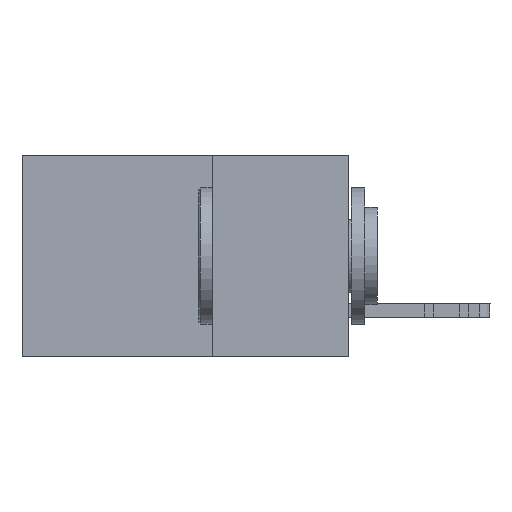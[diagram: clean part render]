
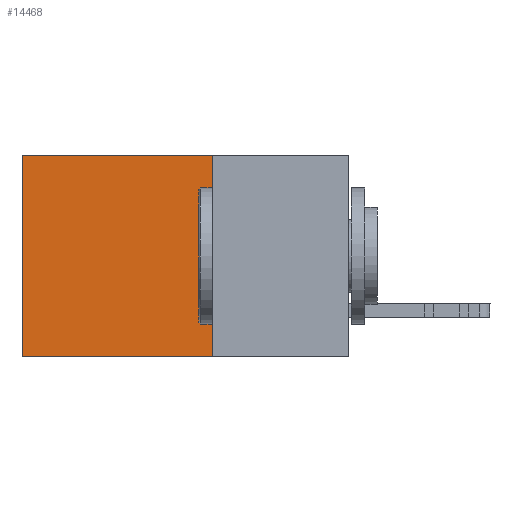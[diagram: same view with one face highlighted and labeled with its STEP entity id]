
A CAD part, left-side view. The second image highlights one B-rep face of the part: STEP entity #14468.
In plain terms, the highlighted planar face has unit normal (-1, 0, 0).
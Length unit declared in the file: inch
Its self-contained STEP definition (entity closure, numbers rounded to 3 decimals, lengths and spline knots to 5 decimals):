
#1124 = VERTEX_POINT ( 'NONE', #23269 ) ;
#1845 = EDGE_CURVE ( 'NONE', #1124, #4888, #21866, .T. ) ;
#1887 = PLANE ( 'NONE',  #4446 ) ;
#2010 = ORIENTED_EDGE ( 'NONE', *, *, #7004, .T. ) ;
#3060 = DIRECTION ( 'NONE',  ( 0., 1., 0. ) ) ;
#3591 = EDGE_CURVE ( 'NONE', #21165, #1124, #6470, .T. ) ;
#3854 = FACE_OUTER_BOUND ( 'NONE', #20830, .T. ) ;
#4355 = CARTESIAN_POINT ( 'NONE',  ( 0.2615, 0.6, 0. ) ) ;
#4446 = AXIS2_PLACEMENT_3D ( 'NONE', #11112, #18379, #12831 ) ;
#4888 = VERTEX_POINT ( 'NONE', #5523 ) ;
#5523 = CARTESIAN_POINT ( 'NONE',  ( 0.2615, 0.6, -0.37 ) ) ;
#6470 = LINE ( 'NONE', #20003, #7364 ) ;
#6588 = DIRECTION ( 'NONE',  ( 0., 0., -1. ) ) ;
#7004 = EDGE_CURVE ( 'NONE', #21165, #9248, #16451, .T. ) ;
#7364 = VECTOR ( 'NONE', #6588, 39.37008 ) ;
#8497 = VECTOR ( 'NONE', #16259, 39.37008 ) ;
#8651 = CARTESIAN_POINT ( 'NONE',  ( 0.2615, 0.6, -0.37 ) ) ;
#9248 = VERTEX_POINT ( 'NONE', #4355 ) ;
#11112 = CARTESIAN_POINT ( 'NONE',  ( 0.2615, 0.25, -0.37 ) ) ;
#12512 = CARTESIAN_POINT ( 'NONE',  ( 0.2615, 0.25, 0. ) ) ;
#12597 = CARTESIAN_POINT ( 'NONE',  ( 0.2615, 0.25, -0.37 ) ) ;
#12831 = DIRECTION ( 'NONE',  ( 0., 0., -1. ) ) ;
#13262 = ORIENTED_EDGE ( 'NONE', *, *, #3591, .F. ) ;
#13678 = CARTESIAN_POINT ( 'NONE',  ( 0.2615, 0.25, 0. ) ) ;
#14468 = ADVANCED_FACE ( 'NONE', ( #3854 ), #1887, .F. ) ;
#15264 = VECTOR ( 'NONE', #3060, 39.37008 ) ;
#16259 = DIRECTION ( 'NONE',  ( 0., 0., -1. ) ) ;
#16451 = LINE ( 'NONE', #12512, #15264 ) ;
#17516 = VECTOR ( 'NONE', #20130, 39.37008 ) ;
#18379 = DIRECTION ( 'NONE',  ( 1., 0., 0. ) ) ;
#20003 = CARTESIAN_POINT ( 'NONE',  ( 0.2615, 0.25, -0.37 ) ) ;
#20130 = DIRECTION ( 'NONE',  ( 0., 1., 0. ) ) ;
#20830 = EDGE_LOOP ( 'NONE', ( #21290, #22391, #13262, #2010 ) ) ;
#21165 = VERTEX_POINT ( 'NONE', #13678 ) ;
#21290 = ORIENTED_EDGE ( 'NONE', *, *, #21292, .T. ) ;
#21292 = EDGE_CURVE ( 'NONE', #9248, #4888, #21701, .T. ) ;
#21701 = LINE ( 'NONE', #8651, #8497 ) ;
#21866 = LINE ( 'NONE', #12597, #17516 ) ;
#22391 = ORIENTED_EDGE ( 'NONE', *, *, #1845, .F. ) ;
#23269 = CARTESIAN_POINT ( 'NONE',  ( 0.2615, 0.25, -0.37 ) ) ;
